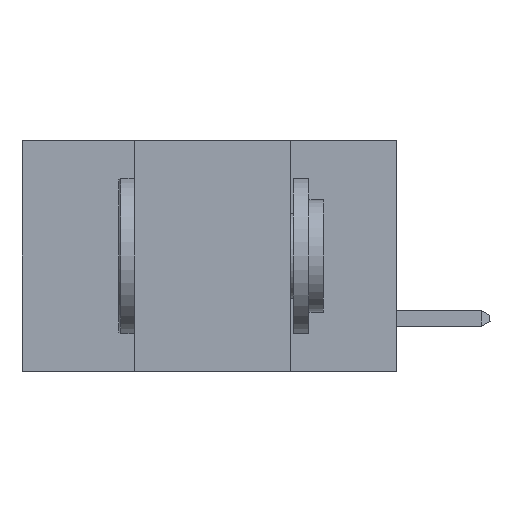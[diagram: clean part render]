
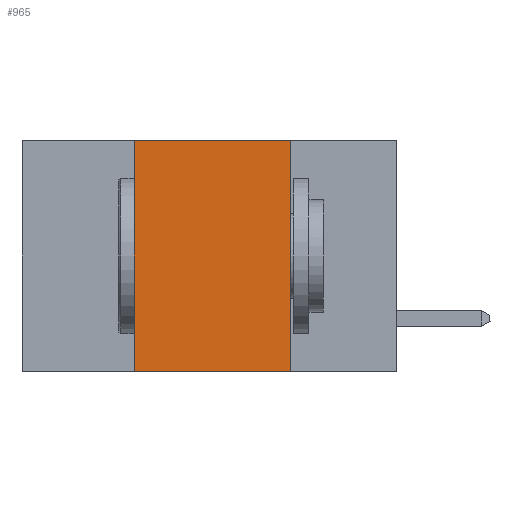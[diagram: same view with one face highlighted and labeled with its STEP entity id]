
A CAD part, left-side view. The second image highlights one B-rep face of the part: STEP entity #965.
In plain terms, the highlighted planar face has unit normal (-1, 0, 0).
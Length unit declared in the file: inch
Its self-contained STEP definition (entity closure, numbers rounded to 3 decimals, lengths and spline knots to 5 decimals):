
#683 = ORIENTED_EDGE ( 'NONE', *, *, #945, .F. ) ;
#880 = VECTOR ( 'NONE', #5805, 39.37008 ) ;
#945 = EDGE_CURVE ( 'NONE', #8073, #9970, #12825, .T. ) ;
#965 = ADVANCED_FACE ( 'NONE', ( #1361 ), #8440, .F. ) ;
#1071 = EDGE_LOOP ( 'NONE', ( #8164, #683, #6078, #3841 ) ) ;
#1361 = FACE_OUTER_BOUND ( 'NONE', #1071, .T. ) ;
#1392 = CARTESIAN_POINT ( 'NONE',  ( 0., 0.17, 0. ) ) ;
#1962 = CARTESIAN_POINT ( 'NONE',  ( 0., 0.6, 0. ) ) ;
#2080 = EDGE_CURVE ( 'NONE', #5385, #7021, #13418, .T. ) ;
#2455 = VECTOR ( 'NONE', #6047, 39.37008 ) ;
#2783 = LINE ( 'NONE', #11210, #2455 ) ;
#3841 = ORIENTED_EDGE ( 'NONE', *, *, #2080, .T. ) ;
#4836 = DIRECTION ( 'NONE',  ( 0., 0., -1. ) ) ;
#5385 = VERTEX_POINT ( 'NONE', #13598 ) ;
#5415 = VECTOR ( 'NONE', #11077, 39.37008 ) ;
#5805 = DIRECTION ( 'NONE',  ( 0., 0., -1. ) ) ;
#6047 = DIRECTION ( 'NONE',  ( 0., 0., 1. ) ) ;
#6078 = ORIENTED_EDGE ( 'NONE', *, *, #12176, .F. ) ;
#6217 = CARTESIAN_POINT ( 'NONE',  ( 0., 0.42, 0. ) ) ;
#6987 = VECTOR ( 'NONE', #9182, 39.37008 ) ;
#7021 = VERTEX_POINT ( 'NONE', #10244 ) ;
#8073 = VERTEX_POINT ( 'NONE', #6217 ) ;
#8164 = ORIENTED_EDGE ( 'NONE', *, *, #10066, .F. ) ;
#8371 = DIRECTION ( 'NONE',  ( 1., 0., 0. ) ) ;
#8440 = PLANE ( 'NONE',  #10052 ) ;
#8671 = LINE ( 'NONE', #9909, #880 ) ;
#9182 = DIRECTION ( 'NONE',  ( 0., -1., 0. ) ) ;
#9909 = CARTESIAN_POINT ( 'NONE',  ( 0., 0.17, 0. ) ) ;
#9970 = VERTEX_POINT ( 'NONE', #1392 ) ;
#9972 = CARTESIAN_POINT ( 'NONE',  ( 0., 0.6, 0. ) ) ;
#10052 = AXIS2_PLACEMENT_3D ( 'NONE', #9972, #8371, #4836 ) ;
#10066 = EDGE_CURVE ( 'NONE', #9970, #7021, #8671, .T. ) ;
#10244 = CARTESIAN_POINT ( 'NONE',  ( 0., 0.17, -0.37 ) ) ;
#11077 = DIRECTION ( 'NONE',  ( 0., -1., 0. ) ) ;
#11210 = CARTESIAN_POINT ( 'NONE',  ( 0., 0.42, 0. ) ) ;
#11956 = CARTESIAN_POINT ( 'NONE',  ( 0., 0.6, -0.37 ) ) ;
#12176 = EDGE_CURVE ( 'NONE', #5385, #8073, #2783, .T. ) ;
#12825 = LINE ( 'NONE', #1962, #6987 ) ;
#13418 = LINE ( 'NONE', #11956, #5415 ) ;
#13598 = CARTESIAN_POINT ( 'NONE',  ( 0., 0.42, -0.37 ) ) ;
